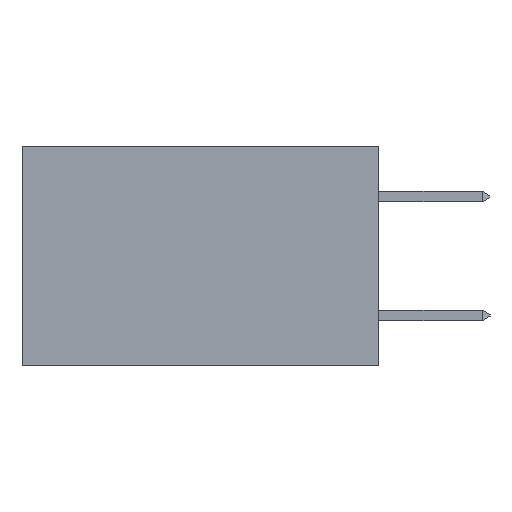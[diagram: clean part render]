
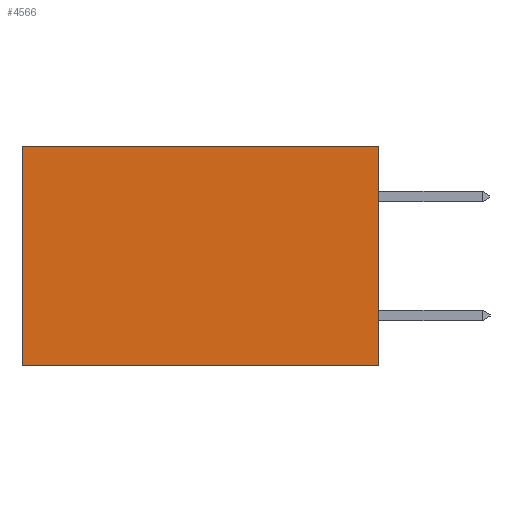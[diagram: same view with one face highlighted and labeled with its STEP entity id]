
A CAD part, left-side view. The second image highlights one B-rep face of the part: STEP entity #4566.
In plain terms, the highlighted planar face has unit normal (-1, 0, 0).
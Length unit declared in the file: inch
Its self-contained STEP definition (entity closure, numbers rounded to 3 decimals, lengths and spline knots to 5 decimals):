
#221 = VECTOR ( 'NONE', #20041, 39.37008 ) ;
#726 = LINE ( 'NONE', #10458, #221 ) ;
#2313 = ORIENTED_EDGE ( 'NONE', *, *, #5296, .T. ) ;
#2964 = VERTEX_POINT ( 'NONE', #20428 ) ;
#3201 = EDGE_CURVE ( 'NONE', #19385, #2964, #13010, .T. ) ;
#3729 = LINE ( 'NONE', #7407, #15562 ) ;
#3850 = EDGE_LOOP ( 'NONE', ( #2313, #12945, #13431, #9930 ) ) ;
#4219 = DIRECTION ( 'NONE',  ( 0., 0., -1. ) ) ;
#4350 = DIRECTION ( 'NONE',  ( 1., 0., 0. ) ) ;
#4389 = VECTOR ( 'NONE', #19938, 39.37008 ) ;
#4566 = ADVANCED_FACE ( 'NONE', ( #12969 ), #4905, .F. ) ;
#4905 = PLANE ( 'NONE',  #8433 ) ;
#4999 = CARTESIAN_POINT ( 'NONE',  ( 0.2615, 0., -0.37 ) ) ;
#5296 = EDGE_CURVE ( 'NONE', #14327, #7297, #6799, .T. ) ;
#5762 = CARTESIAN_POINT ( 'NONE',  ( 0.2615, 0., -0.37 ) ) ;
#6799 = LINE ( 'NONE', #10733, #10622 ) ;
#7297 = VERTEX_POINT ( 'NONE', #18607 ) ;
#7407 = CARTESIAN_POINT ( 'NONE',  ( 0.2615, 0., -0.37 ) ) ;
#8433 = AXIS2_PLACEMENT_3D ( 'NONE', #4999, #4350, #4219 ) ;
#8977 = EDGE_CURVE ( 'NONE', #19385, #14327, #726, .T. ) ;
#9930 = ORIENTED_EDGE ( 'NONE', *, *, #8977, .T. ) ;
#10175 = CARTESIAN_POINT ( 'NONE',  ( 0.2615, 0., 0. ) ) ;
#10458 = CARTESIAN_POINT ( 'NONE',  ( 0.2615, 0., 0. ) ) ;
#10621 = DIRECTION ( 'NONE',  ( 0., 1., 0. ) ) ;
#10622 = VECTOR ( 'NONE', #12396, 39.37008 ) ;
#10733 = CARTESIAN_POINT ( 'NONE',  ( 0.2615, 0.6, -0.37 ) ) ;
#12396 = DIRECTION ( 'NONE',  ( 0., 0., -1. ) ) ;
#12431 = CARTESIAN_POINT ( 'NONE',  ( 0.2615, 0.6, 0. ) ) ;
#12945 = ORIENTED_EDGE ( 'NONE', *, *, #20235, .F. ) ;
#12969 = FACE_OUTER_BOUND ( 'NONE', #3850, .T. ) ;
#13010 = LINE ( 'NONE', #5762, #4389 ) ;
#13431 = ORIENTED_EDGE ( 'NONE', *, *, #3201, .F. ) ;
#14327 = VERTEX_POINT ( 'NONE', #12431 ) ;
#15562 = VECTOR ( 'NONE', #10621, 39.37008 ) ;
#18607 = CARTESIAN_POINT ( 'NONE',  ( 0.2615, 0.6, -0.37 ) ) ;
#19385 = VERTEX_POINT ( 'NONE', #10175 ) ;
#19938 = DIRECTION ( 'NONE',  ( 0., 0., -1. ) ) ;
#20041 = DIRECTION ( 'NONE',  ( 0., 1., 0. ) ) ;
#20235 = EDGE_CURVE ( 'NONE', #2964, #7297, #3729, .T. ) ;
#20428 = CARTESIAN_POINT ( 'NONE',  ( 0.2615, 0., -0.37 ) ) ;
